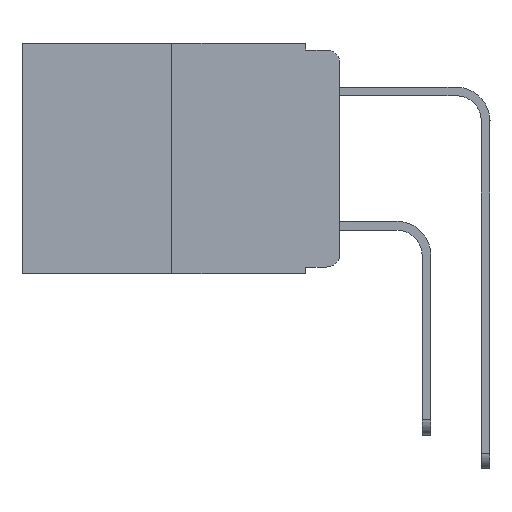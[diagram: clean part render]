
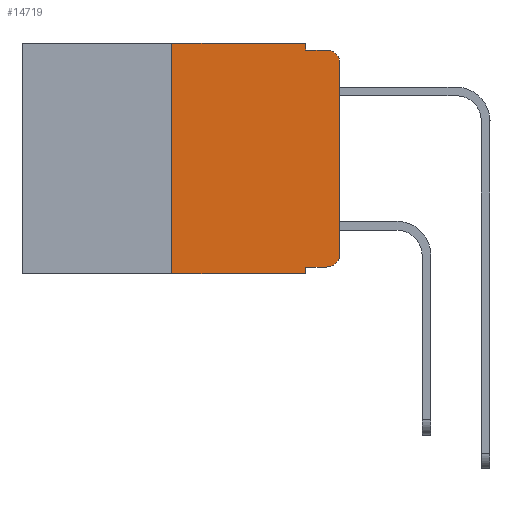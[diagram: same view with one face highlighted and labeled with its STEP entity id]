
A CAD part, left-side view. The second image highlights one B-rep face of the part: STEP entity #14719.
In plain terms, the highlighted planar face has unit normal (-1, 0, 0).
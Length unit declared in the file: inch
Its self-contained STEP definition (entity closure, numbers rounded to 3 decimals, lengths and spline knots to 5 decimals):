
#65 = FACE_OUTER_BOUND ( 'NONE', #24849, .T. ) ;
#112 = DIRECTION ( 'NONE',  ( 0., 0., -1. ) ) ;
#114 = ORIENTED_EDGE ( 'NONE', *, *, #9131, .T. ) ;
#392 = VERTEX_POINT ( 'NONE', #5835 ) ;
#453 = ORIENTED_EDGE ( 'NONE', *, *, #6898, .T. ) ;
#522 = ORIENTED_EDGE ( 'NONE', *, *, #5467, .F. ) ;
#1328 = LINE ( 'NONE', #21112, #25275 ) ;
#1456 = ORIENTED_EDGE ( 'NONE', *, *, #19935, .F. ) ;
#1624 = CARTESIAN_POINT ( 'NONE',  ( 0., 0.051, -0.333 ) ) ;
#1862 = VERTEX_POINT ( 'NONE', #17942 ) ;
#1953 = EDGE_CURVE ( 'NONE', #16422, #392, #17559, .T. ) ;
#2337 = CARTESIAN_POINT ( 'NONE',  ( 0., 0.051, 0. ) ) ;
#2849 = CARTESIAN_POINT ( 'NONE',  ( 0., 0.051, 0. ) ) ;
#4140 = DIRECTION ( 'NONE',  ( 0., -1., 0. ) ) ;
#4159 = VECTOR ( 'NONE', #20141, 39.37008 ) ;
#4591 = DIRECTION ( 'NONE',  ( 0., 0., -1. ) ) ;
#5467 = EDGE_CURVE ( 'NONE', #16422, #1862, #1328, .T. ) ;
#5491 = CARTESIAN_POINT ( 'NONE',  ( 0., 0.051, 0. ) ) ;
#5835 = CARTESIAN_POINT ( 'NONE',  ( 0., 0.051, -0.343 ) ) ;
#5876 = DIRECTION ( 'NONE',  ( 0., 0., 1. ) ) ;
#6244 = VECTOR ( 'NONE', #4140, 39.37008 ) ;
#6325 = CARTESIAN_POINT ( 'NONE',  ( 0., 0.02, -0.03 ) ) ;
#6516 = CARTESIAN_POINT ( 'NONE',  ( 0., 0.473, 0. ) ) ;
#6882 = DIRECTION ( 'NONE',  ( 0., 0., -1. ) ) ;
#6898 = EDGE_CURVE ( 'NONE', #24410, #11341, #23092, .T. ) ;
#7234 = ORIENTED_EDGE ( 'NONE', *, *, #1953, .T. ) ;
#7655 = VECTOR ( 'NONE', #6882, 39.37008 ) ;
#7994 = VERTEX_POINT ( 'NONE', #2337 ) ;
#8375 = DIRECTION ( 'NONE',  ( 0., 0., -1. ) ) ;
#8475 = VECTOR ( 'NONE', #5876, 39.37008 ) ;
#9131 = EDGE_CURVE ( 'NONE', #11341, #21187, #9706, .T. ) ;
#9245 = ORIENTED_EDGE ( 'NONE', *, *, #21834, .T. ) ;
#9706 = CIRCLE ( 'NONE', #11612, 0.02 ) ;
#9788 = CIRCLE ( 'NONE', #25065, 0.02 ) ;
#10443 = ORIENTED_EDGE ( 'NONE', *, *, #22919, .F. ) ;
#10641 = PLANE ( 'NONE',  #13360 ) ;
#11341 = VERTEX_POINT ( 'NONE', #23227 ) ;
#11474 = CARTESIAN_POINT ( 'NONE',  ( 0., 0., -0.03 ) ) ;
#11508 = ORIENTED_EDGE ( 'NONE', *, *, #11986, .F. ) ;
#11612 = AXIS2_PLACEMENT_3D ( 'NONE', #24026, #12290, #112 ) ;
#11930 = DIRECTION ( 'NONE',  ( 0., -1., 0. ) ) ;
#11986 = EDGE_CURVE ( 'NONE', #7994, #18135, #17600, .T. ) ;
#12290 = DIRECTION ( 'NONE',  ( -1., 0., 0. ) ) ;
#12327 = VECTOR ( 'NONE', #21427, 39.37008 ) ;
#12563 = EDGE_CURVE ( 'NONE', #18137, #19067, #9788, .T. ) ;
#13076 = EDGE_CURVE ( 'NONE', #18135, #19067, #14435, .T. ) ;
#13201 = DIRECTION ( 'NONE',  ( 0., 0., 1. ) ) ;
#13360 = AXIS2_PLACEMENT_3D ( 'NONE', #6516, #16595, #4591 ) ;
#14435 = LINE ( 'NONE', #19876, #24201 ) ;
#14719 = ADVANCED_FACE ( 'NONE', ( #65 ), #10641, .F. ) ;
#14830 = LINE ( 'NONE', #18164, #4159 ) ;
#15668 = ORIENTED_EDGE ( 'NONE', *, *, #12563, .T. ) ;
#15698 = DIRECTION ( 'NONE',  ( 0., -1., 0. ) ) ;
#15882 = CARTESIAN_POINT ( 'NONE',  ( 0., 0., 0. ) ) ;
#16422 = VERTEX_POINT ( 'NONE', #22556 ) ;
#16595 = DIRECTION ( 'NONE',  ( 1., 0., 0. ) ) ;
#17403 = ORIENTED_EDGE ( 'NONE', *, *, #13076, .F. ) ;
#17559 = LINE ( 'NONE', #21569, #6244 ) ;
#17600 = LINE ( 'NONE', #5491, #12327 ) ;
#17834 = CARTESIAN_POINT ( 'NONE',  ( 0., 0., -0.313 ) ) ;
#17920 = VECTOR ( 'NONE', #15698, 39.37008 ) ;
#17942 = CARTESIAN_POINT ( 'NONE',  ( 0., 0.25, 0. ) ) ;
#18135 = VERTEX_POINT ( 'NONE', #23228 ) ;
#18137 = VERTEX_POINT ( 'NONE', #11474 ) ;
#18164 = CARTESIAN_POINT ( 'NONE',  ( 0., 0.473, 0. ) ) ;
#18285 = LINE ( 'NONE', #2849, #7655 ) ;
#19067 = VERTEX_POINT ( 'NONE', #24168 ) ;
#19876 = CARTESIAN_POINT ( 'NONE',  ( 0., 0.051, -0.01 ) ) ;
#19935 = EDGE_CURVE ( 'NONE', #24410, #392, #18285, .T. ) ;
#20141 = DIRECTION ( 'NONE',  ( 0., -1., 0. ) ) ;
#20298 = DIRECTION ( 'NONE',  ( -1., 0., 0. ) ) ;
#20917 = LINE ( 'NONE', #15882, #8475 ) ;
#21112 = CARTESIAN_POINT ( 'NONE',  ( 0., 0.25, 0. ) ) ;
#21187 = VERTEX_POINT ( 'NONE', #17834 ) ;
#21427 = DIRECTION ( 'NONE',  ( 0., 0., -1. ) ) ;
#21569 = CARTESIAN_POINT ( 'NONE',  ( 0., 0.473, -0.343 ) ) ;
#21834 = EDGE_CURVE ( 'NONE', #21187, #18137, #20917, .T. ) ;
#22556 = CARTESIAN_POINT ( 'NONE',  ( 0., 0.25, -0.343 ) ) ;
#22919 = EDGE_CURVE ( 'NONE', #1862, #7994, #14830, .T. ) ;
#23092 = LINE ( 'NONE', #1624, #17920 ) ;
#23227 = CARTESIAN_POINT ( 'NONE',  ( 0., 0.02, -0.333 ) ) ;
#23228 = CARTESIAN_POINT ( 'NONE',  ( 0., 0.051, -0.01 ) ) ;
#24026 = CARTESIAN_POINT ( 'NONE',  ( 0., 0.02, -0.313 ) ) ;
#24168 = CARTESIAN_POINT ( 'NONE',  ( 0., 0.02, -0.01 ) ) ;
#24201 = VECTOR ( 'NONE', #11930, 39.37008 ) ;
#24410 = VERTEX_POINT ( 'NONE', #25042 ) ;
#24849 = EDGE_LOOP ( 'NONE', ( #9245, #15668, #17403, #11508, #10443, #522, #7234, #1456, #453, #114 ) ) ;
#25042 = CARTESIAN_POINT ( 'NONE',  ( 0., 0.051, -0.333 ) ) ;
#25065 = AXIS2_PLACEMENT_3D ( 'NONE', #6325, #20298, #8375 ) ;
#25275 = VECTOR ( 'NONE', #13201, 39.37008 ) ;
